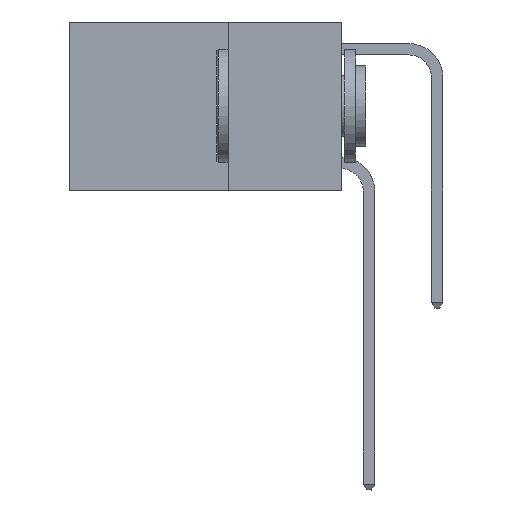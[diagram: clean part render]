
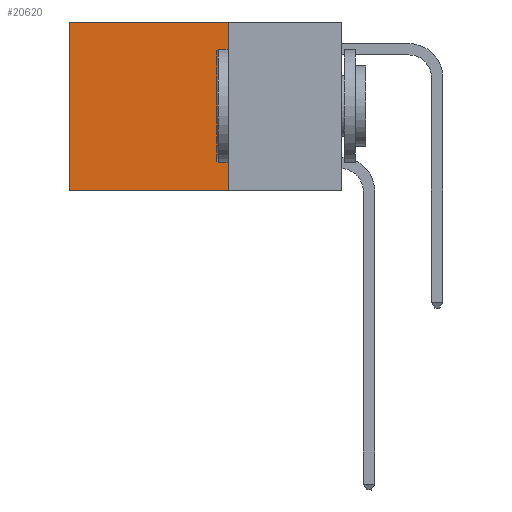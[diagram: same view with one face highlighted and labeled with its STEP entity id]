
A CAD part, left-side view. The second image highlights one B-rep face of the part: STEP entity #20620.
In plain terms, the highlighted planar face has unit normal (-1, 0, 0).
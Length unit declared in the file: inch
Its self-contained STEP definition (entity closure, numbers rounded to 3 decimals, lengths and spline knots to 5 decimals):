
#933 = CARTESIAN_POINT ( 'NONE',  ( 0.2625, 0.25, -0.37 ) ) ;
#1123 = PLANE ( 'NONE',  #11061 ) ;
#1804 = VERTEX_POINT ( 'NONE', #21789 ) ;
#1855 = LINE ( 'NONE', #16383, #13682 ) ;
#2441 = VECTOR ( 'NONE', #5978, 39.37008 ) ;
#3394 = DIRECTION ( 'NONE',  ( 1., 0., 0. ) ) ;
#3781 = EDGE_CURVE ( 'NONE', #1804, #10327, #1855, .T. ) ;
#4278 = CARTESIAN_POINT ( 'NONE',  ( 0.2625, 0.6, 0. ) ) ;
#4736 = EDGE_LOOP ( 'NONE', ( #24403, #24230, #21885, #8975 ) ) ;
#5978 = DIRECTION ( 'NONE',  ( 0., 1., 0. ) ) ;
#8975 = ORIENTED_EDGE ( 'NONE', *, *, #21278, .T. ) ;
#9919 = CARTESIAN_POINT ( 'NONE',  ( 0.2625, 0.25, 0. ) ) ;
#10140 = LINE ( 'NONE', #11627, #26000 ) ;
#10327 = VERTEX_POINT ( 'NONE', #933 ) ;
#10807 = EDGE_CURVE ( 'NONE', #13841, #20948, #25262, .T. ) ;
#11061 = AXIS2_PLACEMENT_3D ( 'NONE', #9919, #3394, #22111 ) ;
#11196 = CARTESIAN_POINT ( 'NONE',  ( 0.2625, 0.6, 0. ) ) ;
#11627 = CARTESIAN_POINT ( 'NONE',  ( 0.2625, 0.25, -0.37 ) ) ;
#11883 = EDGE_CURVE ( 'NONE', #10327, #20948, #10140, .T. ) ;
#12470 = CARTESIAN_POINT ( 'NONE',  ( 0.2625, 0.25, 0. ) ) ;
#13013 = CARTESIAN_POINT ( 'NONE',  ( 0.2625, 0.6, -0.37 ) ) ;
#13682 = VECTOR ( 'NONE', #22581, 39.37008 ) ;
#13841 = VERTEX_POINT ( 'NONE', #4278 ) ;
#13917 = DIRECTION ( 'NONE',  ( 0., 1., 0. ) ) ;
#16383 = CARTESIAN_POINT ( 'NONE',  ( 0.2625, 0.25, 0. ) ) ;
#17930 = DIRECTION ( 'NONE',  ( 0., 0., -1. ) ) ;
#20620 = ADVANCED_FACE ( 'NONE', ( #25745 ), #1123, .F. ) ;
#20948 = VERTEX_POINT ( 'NONE', #13013 ) ;
#21278 = EDGE_CURVE ( 'NONE', #1804, #13841, #24783, .T. ) ;
#21789 = CARTESIAN_POINT ( 'NONE',  ( 0.2625, 0.25, 0. ) ) ;
#21885 = ORIENTED_EDGE ( 'NONE', *, *, #3781, .F. ) ;
#22111 = DIRECTION ( 'NONE',  ( 0., 0., -1. ) ) ;
#22301 = VECTOR ( 'NONE', #17930, 39.37008 ) ;
#22581 = DIRECTION ( 'NONE',  ( 0., 0., -1. ) ) ;
#24230 = ORIENTED_EDGE ( 'NONE', *, *, #11883, .F. ) ;
#24403 = ORIENTED_EDGE ( 'NONE', *, *, #10807, .T. ) ;
#24783 = LINE ( 'NONE', #12470, #2441 ) ;
#25262 = LINE ( 'NONE', #11196, #22301 ) ;
#25745 = FACE_OUTER_BOUND ( 'NONE', #4736, .T. ) ;
#26000 = VECTOR ( 'NONE', #13917, 39.37008 ) ;
